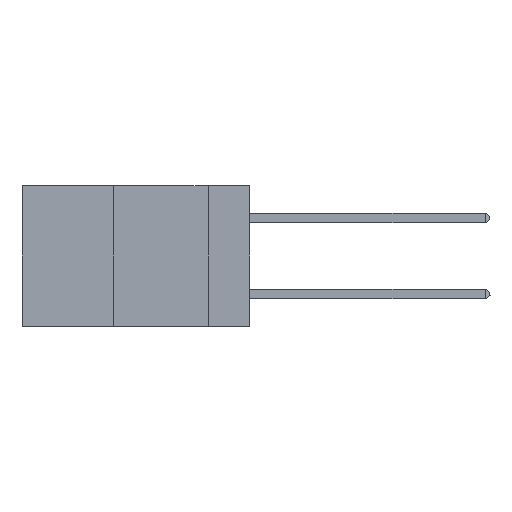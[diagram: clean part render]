
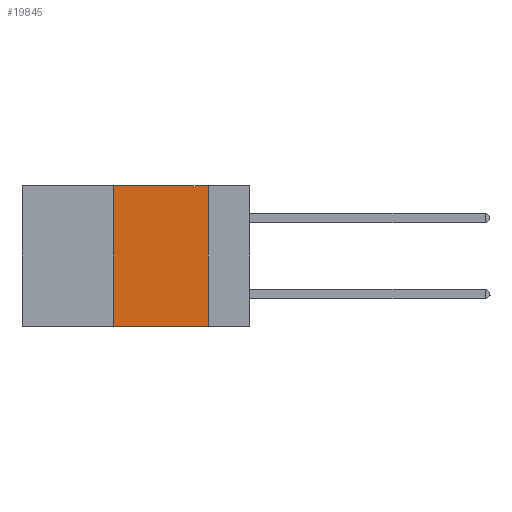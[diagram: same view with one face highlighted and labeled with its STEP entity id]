
A CAD part, left-side view. The second image highlights one B-rep face of the part: STEP entity #19845.
In plain terms, the highlighted planar face has unit normal (-1, 0, 0).
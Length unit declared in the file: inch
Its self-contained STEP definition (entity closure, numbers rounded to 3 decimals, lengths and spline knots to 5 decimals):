
#1950 = CARTESIAN_POINT ( 'NONE',  ( 0., 0.11, 0. ) ) ;
#2699 = VERTEX_POINT ( 'NONE', #35681 ) ;
#2746 = VERTEX_POINT ( 'NONE', #31519 ) ;
#2790 = LINE ( 'NONE', #20174, #21628 ) ;
#2939 = CARTESIAN_POINT ( 'NONE',  ( 0., 0.6, 0. ) ) ;
#3705 = FACE_OUTER_BOUND ( 'NONE', #7154, .T. ) ;
#5280 = LINE ( 'NONE', #25657, #36643 ) ;
#6428 = VECTOR ( 'NONE', #11195, 39.37008 ) ;
#6773 = EDGE_CURVE ( 'NONE', #24504, #33541, #11061, .T. ) ;
#7154 = EDGE_LOOP ( 'NONE', ( #32212, #31037, #36175, #32885 ) ) ;
#8377 = PLANE ( 'NONE',  #26232 ) ;
#11061 = LINE ( 'NONE', #2939, #6428 ) ;
#11195 = DIRECTION ( 'NONE',  ( 0., -1., 0. ) ) ;
#13827 = VECTOR ( 'NONE', #22602, 39.37008 ) ;
#15633 = LINE ( 'NONE', #1950, #13827 ) ;
#16632 = DIRECTION ( 'NONE',  ( 0., 0., 1. ) ) ;
#17133 = DIRECTION ( 'NONE',  ( 0., 0., -1. ) ) ;
#19845 = ADVANCED_FACE ( 'NONE', ( #3705 ), #8377, .F. ) ;
#20159 = CARTESIAN_POINT ( 'NONE',  ( 0., 0.36, 0. ) ) ;
#20174 = CARTESIAN_POINT ( 'NONE',  ( 0., 0.6, -0.37 ) ) ;
#21628 = VECTOR ( 'NONE', #32210, 39.37008 ) ;
#22602 = DIRECTION ( 'NONE',  ( 0., 0., -1. ) ) ;
#24504 = VERTEX_POINT ( 'NONE', #20159 ) ;
#25657 = CARTESIAN_POINT ( 'NONE',  ( 0., 0.36, 0. ) ) ;
#26232 = AXIS2_PLACEMENT_3D ( 'NONE', #37648, #34841, #17133 ) ;
#30642 = EDGE_CURVE ( 'NONE', #2746, #2699, #2790, .T. ) ;
#31037 = ORIENTED_EDGE ( 'NONE', *, *, #6773, .F. ) ;
#31519 = CARTESIAN_POINT ( 'NONE',  ( 0., 0.36, -0.37 ) ) ;
#31555 = EDGE_CURVE ( 'NONE', #33541, #2699, #15633, .T. ) ;
#32210 = DIRECTION ( 'NONE',  ( 0., -1., 0. ) ) ;
#32212 = ORIENTED_EDGE ( 'NONE', *, *, #31555, .F. ) ;
#32885 = ORIENTED_EDGE ( 'NONE', *, *, #30642, .T. ) ;
#33541 = VERTEX_POINT ( 'NONE', #37315 ) ;
#34200 = EDGE_CURVE ( 'NONE', #2746, #24504, #5280, .T. ) ;
#34841 = DIRECTION ( 'NONE',  ( 1., 0., 0. ) ) ;
#35681 = CARTESIAN_POINT ( 'NONE',  ( 0., 0.11, -0.37 ) ) ;
#36175 = ORIENTED_EDGE ( 'NONE', *, *, #34200, .F. ) ;
#36643 = VECTOR ( 'NONE', #16632, 39.37008 ) ;
#37315 = CARTESIAN_POINT ( 'NONE',  ( 0., 0.11, 0. ) ) ;
#37648 = CARTESIAN_POINT ( 'NONE',  ( 0., 0.6, 0. ) ) ;
